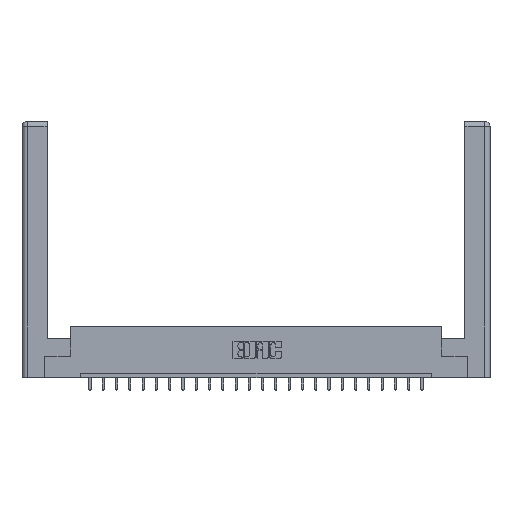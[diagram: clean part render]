
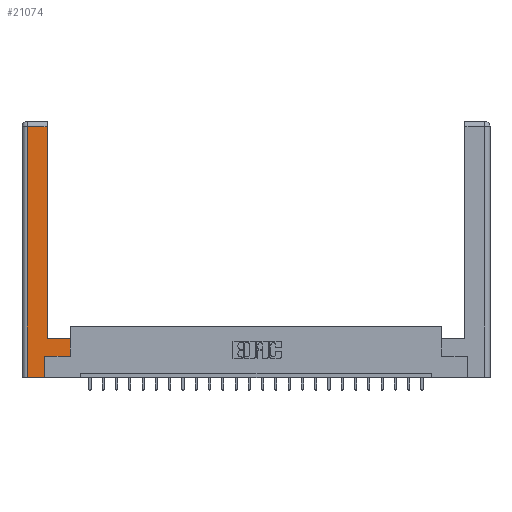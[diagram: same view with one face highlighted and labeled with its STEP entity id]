
A CAD part, top view. The second image highlights one B-rep face of the part: STEP entity #21074.
In plain terms, the highlighted planar face has unit normal (0, 0, 1).
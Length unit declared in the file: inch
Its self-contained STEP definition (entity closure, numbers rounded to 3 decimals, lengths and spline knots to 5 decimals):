
#1156 = PLANE ( 'NONE',  #18188 ) ;
#1439 = ORIENTED_EDGE ( 'NONE', *, *, #18882, .T. ) ;
#2359 = VECTOR ( 'NONE', #12707, 39.37008 ) ;
#2499 = DIRECTION ( 'NONE',  ( 0., 1., 0. ) ) ;
#3037 = VERTEX_POINT ( 'NONE', #17730 ) ;
#3562 = DIRECTION ( 'NONE',  ( 0., 1., 0. ) ) ;
#3773 = LINE ( 'NONE', #23147, #11323 ) ;
#4677 = EDGE_CURVE ( 'NONE', #9219, #20790, #6018, .T. ) ;
#5300 = LINE ( 'NONE', #15529, #13097 ) ;
#5682 = ORIENTED_EDGE ( 'NONE', *, *, #4677, .T. ) ;
#6018 = LINE ( 'NONE', #6118, #19357 ) ;
#6118 = CARTESIAN_POINT ( 'NONE',  ( 0.265, 0.245, 0. ) ) ;
#6760 = CARTESIAN_POINT ( 'NONE',  ( 0.0615, 0., 0. ) ) ;
#6791 = LINE ( 'NONE', #11911, #16376 ) ;
#7012 = VERTEX_POINT ( 'NONE', #13063 ) ;
#7960 = DIRECTION ( 'NONE',  ( 0., 1., 0. ) ) ;
#8029 = CARTESIAN_POINT ( 'NONE',  ( 0.565, 0.45, 0. ) ) ;
#8346 = EDGE_CURVE ( 'NONE', #16782, #12486, #18449, .T. ) ;
#8901 = EDGE_CURVE ( 'NONE', #7012, #16782, #6791, .T. ) ;
#9219 = VERTEX_POINT ( 'NONE', #13119 ) ;
#9564 = LINE ( 'NONE', #8029, #22068 ) ;
#9898 = DIRECTION ( 'NONE',  ( -1., 0., 0. ) ) ;
#10259 = ORIENTED_EDGE ( 'NONE', *, *, #8901, .T. ) ;
#10846 = CARTESIAN_POINT ( 'NONE',  ( 0.295, 0.45, 0. ) ) ;
#11107 = CARTESIAN_POINT ( 'NONE',  ( 0.295, 3., 0. ) ) ;
#11323 = VECTOR ( 'NONE', #12033, 39.37008 ) ;
#11626 = CARTESIAN_POINT ( 'NONE',  ( 0.265, 0.245, 0. ) ) ;
#11911 = CARTESIAN_POINT ( 'NONE',  ( 0.0615, 2.94, 0. ) ) ;
#12033 = DIRECTION ( 'NONE',  ( 1., 0., 0. ) ) ;
#12065 = VERTEX_POINT ( 'NONE', #19818 ) ;
#12486 = VERTEX_POINT ( 'NONE', #6760 ) ;
#12707 = DIRECTION ( 'NONE',  ( -1., 0., 0. ) ) ;
#13063 = CARTESIAN_POINT ( 'NONE',  ( 0.295, 2.94, 0. ) ) ;
#13097 = VECTOR ( 'NONE', #18846, 39.37008 ) ;
#13119 = CARTESIAN_POINT ( 'NONE',  ( 0.265, 0., 0. ) ) ;
#13721 = DIRECTION ( 'NONE',  ( 0., -1., 0. ) ) ;
#14076 = CARTESIAN_POINT ( 'NONE',  ( 0., 0., 0. ) ) ;
#14160 = VERTEX_POINT ( 'NONE', #20565 ) ;
#14237 = DIRECTION ( 'NONE',  ( 0., 0., -1. ) ) ;
#14571 = ORIENTED_EDGE ( 'NONE', *, *, #19645, .T. ) ;
#14675 = ORIENTED_EDGE ( 'NONE', *, *, #19251, .T. ) ;
#14838 = EDGE_CURVE ( 'NONE', #3037, #7012, #21709, .T. ) ;
#15529 = CARTESIAN_POINT ( 'NONE',  ( 0.265, 0., 0. ) ) ;
#16257 = ORIENTED_EDGE ( 'NONE', *, *, #14838, .T. ) ;
#16376 = VECTOR ( 'NONE', #9898, 39.37008 ) ;
#16773 = VECTOR ( 'NONE', #3562, 39.37008 ) ;
#16782 = VERTEX_POINT ( 'NONE', #24014 ) ;
#17311 = CARTESIAN_POINT ( 'NONE',  ( 0.0615, 0., 0. ) ) ;
#17730 = CARTESIAN_POINT ( 'NONE',  ( 0.295, 0.45, 0. ) ) ;
#17783 = EDGE_LOOP ( 'NONE', ( #16257, #10259, #21073, #19124, #5682, #1439, #14675, #14571 ) ) ;
#18188 = AXIS2_PLACEMENT_3D ( 'NONE', #14076, #14237, #21539 ) ;
#18423 = FACE_OUTER_BOUND ( 'NONE', #17783, .T. ) ;
#18449 = LINE ( 'NONE', #17311, #21026 ) ;
#18846 = DIRECTION ( 'NONE',  ( 1., 0., 0. ) ) ;
#18882 = EDGE_CURVE ( 'NONE', #20790, #14160, #3773, .T. ) ;
#19124 = ORIENTED_EDGE ( 'NONE', *, *, #22273, .T. ) ;
#19251 = EDGE_CURVE ( 'NONE', #14160, #12065, #9564, .T. ) ;
#19357 = VECTOR ( 'NONE', #7960, 39.37008 ) ;
#19645 = EDGE_CURVE ( 'NONE', #12065, #3037, #20421, .T. ) ;
#19818 = CARTESIAN_POINT ( 'NONE',  ( 0.565, 0.45, 0. ) ) ;
#20421 = LINE ( 'NONE', #10846, #2359 ) ;
#20565 = CARTESIAN_POINT ( 'NONE',  ( 0.565, 0.245, 0. ) ) ;
#20790 = VERTEX_POINT ( 'NONE', #11626 ) ;
#21026 = VECTOR ( 'NONE', #13721, 39.37008 ) ;
#21073 = ORIENTED_EDGE ( 'NONE', *, *, #8346, .T. ) ;
#21074 = ADVANCED_FACE ( 'NONE', ( #18423 ), #1156, .F. ) ;
#21539 = DIRECTION ( 'NONE',  ( -1., 0., 0. ) ) ;
#21709 = LINE ( 'NONE', #11107, #16773 ) ;
#22068 = VECTOR ( 'NONE', #2499, 39.37008 ) ;
#22273 = EDGE_CURVE ( 'NONE', #12486, #9219, #5300, .T. ) ;
#23147 = CARTESIAN_POINT ( 'NONE',  ( 0.565, 0.245, 0. ) ) ;
#24014 = CARTESIAN_POINT ( 'NONE',  ( 0.0615, 2.94, 0. ) ) ;
